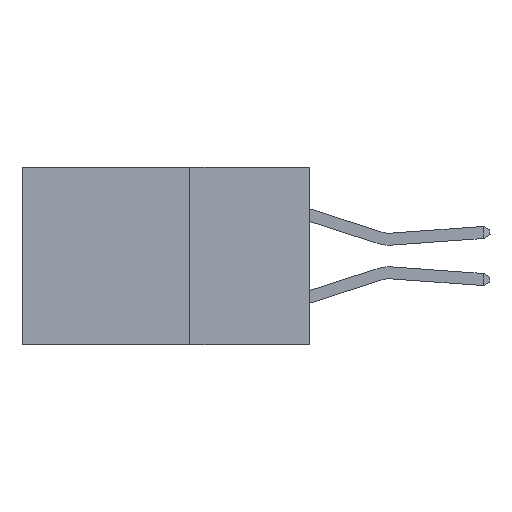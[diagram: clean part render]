
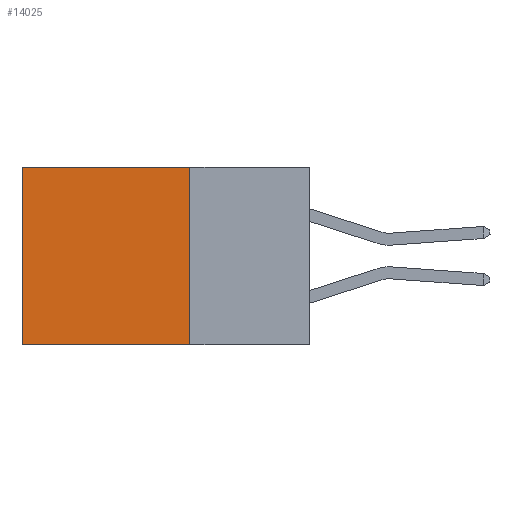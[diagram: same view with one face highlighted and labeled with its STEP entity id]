
A CAD part, left-side view. The second image highlights one B-rep face of the part: STEP entity #14025.
In plain terms, the highlighted planar face has unit normal (-1, 0, 0).
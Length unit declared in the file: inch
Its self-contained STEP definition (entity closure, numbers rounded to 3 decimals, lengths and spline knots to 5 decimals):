
#15 = DIRECTION ( 'NONE',  ( 0., 0., -1. ) ) ;
#98 = VERTEX_POINT ( 'NONE', #13125 ) ;
#271 = CARTESIAN_POINT ( 'NONE',  ( 0.2615, 0.25, -0.37 ) ) ;
#298 = EDGE_CURVE ( 'NONE', #5842, #5143, #1070, .T. ) ;
#644 = DIRECTION ( 'NONE',  ( 1., 0., 0. ) ) ;
#723 = FACE_OUTER_BOUND ( 'NONE', #12521, .T. ) ;
#1070 = LINE ( 'NONE', #6556, #1711 ) ;
#1130 = VECTOR ( 'NONE', #15, 39.37008 ) ;
#1360 = ORIENTED_EDGE ( 'NONE', *, *, #5573, .T. ) ;
#1447 = VECTOR ( 'NONE', #11709, 39.37008 ) ;
#1711 = VECTOR ( 'NONE', #5669, 39.37008 ) ;
#2128 = ORIENTED_EDGE ( 'NONE', *, *, #13910, .F. ) ;
#3234 = CARTESIAN_POINT ( 'NONE',  ( 0.2615, 0.6, 0. ) ) ;
#3349 = EDGE_CURVE ( 'NONE', #98, #3500, #14737, .T. ) ;
#3500 = VERTEX_POINT ( 'NONE', #13896 ) ;
#4937 = ORIENTED_EDGE ( 'NONE', *, *, #3349, .F. ) ;
#5143 = VERTEX_POINT ( 'NONE', #3234 ) ;
#5573 = EDGE_CURVE ( 'NONE', #5143, #3500, #9298, .T. ) ;
#5624 = CARTESIAN_POINT ( 'NONE',  ( 0.2615, 0.25, -0.37 ) ) ;
#5663 = ORIENTED_EDGE ( 'NONE', *, *, #298, .T. ) ;
#5669 = DIRECTION ( 'NONE',  ( 0., 1., 0. ) ) ;
#5842 = VERTEX_POINT ( 'NONE', #6684 ) ;
#5967 = LINE ( 'NONE', #271, #1447 ) ;
#6265 = DIRECTION ( 'NONE',  ( 0., 0., -1. ) ) ;
#6556 = CARTESIAN_POINT ( 'NONE',  ( 0.2615, 0.25, 0. ) ) ;
#6684 = CARTESIAN_POINT ( 'NONE',  ( 0.2615, 0.25, 0. ) ) ;
#8975 = DIRECTION ( 'NONE',  ( 0., 1., 0. ) ) ;
#9298 = LINE ( 'NONE', #13873, #1130 ) ;
#11275 = AXIS2_PLACEMENT_3D ( 'NONE', #12155, #644, #6265 ) ;
#11709 = DIRECTION ( 'NONE',  ( 0., 0., -1. ) ) ;
#12155 = CARTESIAN_POINT ( 'NONE',  ( 0.2615, 0.25, -0.37 ) ) ;
#12521 = EDGE_LOOP ( 'NONE', ( #1360, #4937, #2128, #5663 ) ) ;
#12634 = VECTOR ( 'NONE', #8975, 39.37008 ) ;
#13125 = CARTESIAN_POINT ( 'NONE',  ( 0.2615, 0.25, -0.37 ) ) ;
#13873 = CARTESIAN_POINT ( 'NONE',  ( 0.2615, 0.6, -0.37 ) ) ;
#13896 = CARTESIAN_POINT ( 'NONE',  ( 0.2615, 0.6, -0.37 ) ) ;
#13910 = EDGE_CURVE ( 'NONE', #5842, #98, #5967, .T. ) ;
#14025 = ADVANCED_FACE ( 'NONE', ( #723 ), #14430, .F. ) ;
#14430 = PLANE ( 'NONE',  #11275 ) ;
#14737 = LINE ( 'NONE', #5624, #12634 ) ;
